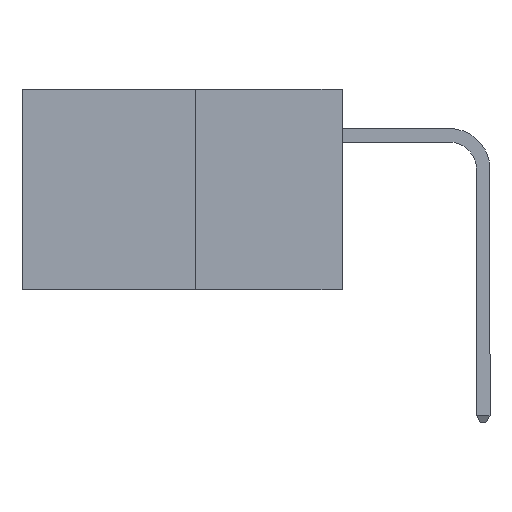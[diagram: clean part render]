
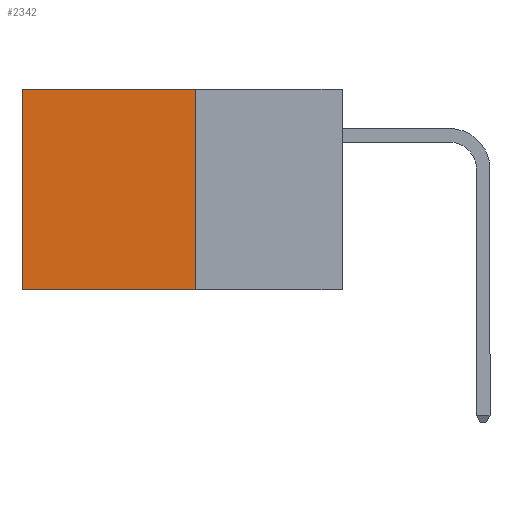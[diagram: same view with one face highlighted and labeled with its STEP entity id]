
A CAD part, left-side view. The second image highlights one B-rep face of the part: STEP entity #2342.
In plain terms, the highlighted planar face has unit normal (-1, 0, 0).
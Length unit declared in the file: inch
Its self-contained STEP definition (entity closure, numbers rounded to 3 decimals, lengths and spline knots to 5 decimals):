
#135 = LINE ( 'NONE', #3981, #7596 ) ;
#587 = VERTEX_POINT ( 'NONE', #1919 ) ;
#1136 = CARTESIAN_POINT ( 'NONE',  ( 0.277, 0.27, -0.37 ) ) ;
#1146 = DIRECTION ( 'NONE',  ( 0., 1., 0. ) ) ;
#1726 = CARTESIAN_POINT ( 'NONE',  ( 0.277, 0.27, 0. ) ) ;
#1919 = CARTESIAN_POINT ( 'NONE',  ( 0.277, 0.59, 0. ) ) ;
#2003 = EDGE_CURVE ( 'NONE', #7458, #7764, #3642, .T. ) ;
#2037 = DIRECTION ( 'NONE',  ( 1., 0., 0. ) ) ;
#2321 = ORIENTED_EDGE ( 'NONE', *, *, #3777, .T. ) ;
#2342 = ADVANCED_FACE ( 'NONE', ( #2590 ), #9197, .F. ) ;
#2590 = FACE_OUTER_BOUND ( 'NONE', #2842, .T. ) ;
#2842 = EDGE_LOOP ( 'NONE', ( #6689, #3337, #5939, #2321 ) ) ;
#3337 = ORIENTED_EDGE ( 'NONE', *, *, #5076, .F. ) ;
#3642 = LINE ( 'NONE', #8296, #5379 ) ;
#3688 = DIRECTION ( 'NONE',  ( 0., 0., -1. ) ) ;
#3694 = DIRECTION ( 'NONE',  ( 0., 0., -1. ) ) ;
#3777 = EDGE_CURVE ( 'NONE', #7458, #587, #7349, .T. ) ;
#3981 = CARTESIAN_POINT ( 'NONE',  ( 0.277, 0.59, -0.37 ) ) ;
#4058 = VECTOR ( 'NONE', #1146, 39.37008 ) ;
#4890 = DIRECTION ( 'NONE',  ( 0., 0., -1. ) ) ;
#5076 = EDGE_CURVE ( 'NONE', #7764, #6697, #5976, .T. ) ;
#5205 = CARTESIAN_POINT ( 'NONE',  ( 0.277, 0.59, -0.37 ) ) ;
#5379 = VECTOR ( 'NONE', #3688, 39.37008 ) ;
#5555 = VECTOR ( 'NONE', #6608, 39.37008 ) ;
#5558 = CARTESIAN_POINT ( 'NONE',  ( 0.277, 0.27, -0.37 ) ) ;
#5939 = ORIENTED_EDGE ( 'NONE', *, *, #2003, .F. ) ;
#5976 = LINE ( 'NONE', #1136, #4058 ) ;
#6608 = DIRECTION ( 'NONE',  ( 0., 1., 0. ) ) ;
#6689 = ORIENTED_EDGE ( 'NONE', *, *, #8318, .T. ) ;
#6697 = VERTEX_POINT ( 'NONE', #5205 ) ;
#7349 = LINE ( 'NONE', #9252, #5555 ) ;
#7458 = VERTEX_POINT ( 'NONE', #1726 ) ;
#7596 = VECTOR ( 'NONE', #3694, 39.37008 ) ;
#7764 = VERTEX_POINT ( 'NONE', #7971 ) ;
#7776 = AXIS2_PLACEMENT_3D ( 'NONE', #5558, #2037, #4890 ) ;
#7971 = CARTESIAN_POINT ( 'NONE',  ( 0.277, 0.27, -0.37 ) ) ;
#8296 = CARTESIAN_POINT ( 'NONE',  ( 0.277, 0.27, -0.37 ) ) ;
#8318 = EDGE_CURVE ( 'NONE', #587, #6697, #135, .T. ) ;
#9197 = PLANE ( 'NONE',  #7776 ) ;
#9252 = CARTESIAN_POINT ( 'NONE',  ( 0.277, 0.27, 0. ) ) ;
